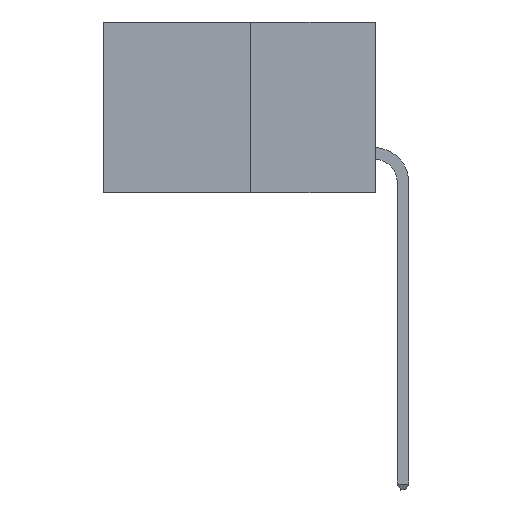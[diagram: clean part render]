
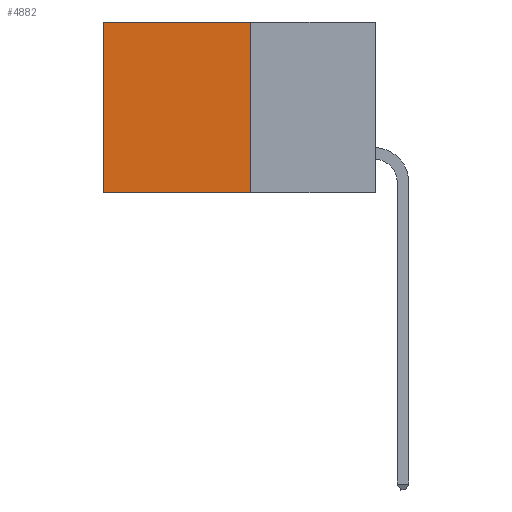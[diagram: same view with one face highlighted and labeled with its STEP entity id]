
A CAD part, left-side view. The second image highlights one B-rep face of the part: STEP entity #4882.
In plain terms, the highlighted planar face has unit normal (-1, 0, 0).
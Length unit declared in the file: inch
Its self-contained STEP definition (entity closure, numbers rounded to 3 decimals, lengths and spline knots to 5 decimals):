
#921 = CARTESIAN_POINT ( 'NONE',  ( 0.277, 0.27, -0.37 ) ) ;
#2353 = EDGE_LOOP ( 'NONE', ( #15523, #5587, #10960, #3823 ) ) ;
#2365 = CARTESIAN_POINT ( 'NONE',  ( 0.277, 0.27, -0.37 ) ) ;
#2819 = CARTESIAN_POINT ( 'NONE',  ( 0.277, 0.59, -0.37 ) ) ;
#2908 = VECTOR ( 'NONE', #8524, 39.37008 ) ;
#3176 = VECTOR ( 'NONE', #13594, 39.37008 ) ;
#3602 = LINE ( 'NONE', #15905, #3176 ) ;
#3663 = PLANE ( 'NONE',  #10400 ) ;
#3823 = ORIENTED_EDGE ( 'NONE', *, *, #6637, .T. ) ;
#3831 = CARTESIAN_POINT ( 'NONE',  ( 0.277, 0.27, -0.37 ) ) ;
#4474 = EDGE_CURVE ( 'NONE', #12852, #8963, #8583, .T. ) ;
#4534 = VECTOR ( 'NONE', #15949, 39.37008 ) ;
#4882 = ADVANCED_FACE ( 'NONE', ( #5289 ), #3663, .F. ) ;
#5234 = LINE ( 'NONE', #5258, #8136 ) ;
#5258 = CARTESIAN_POINT ( 'NONE',  ( 0.277, 0.27, -0.37 ) ) ;
#5289 = FACE_OUTER_BOUND ( 'NONE', #2353, .T. ) ;
#5308 = DIRECTION ( 'NONE',  ( 0., 0., -1. ) ) ;
#5587 = ORIENTED_EDGE ( 'NONE', *, *, #4474, .F. ) ;
#6637 = EDGE_CURVE ( 'NONE', #14142, #12935, #3602, .T. ) ;
#7026 = CARTESIAN_POINT ( 'NONE',  ( 0.277, 0.27, 0. ) ) ;
#7320 = CARTESIAN_POINT ( 'NONE',  ( 0.277, 0.59, -0.37 ) ) ;
#7426 = DIRECTION ( 'NONE',  ( 1., 0., 0. ) ) ;
#8136 = VECTOR ( 'NONE', #5308, 39.37008 ) ;
#8376 = EDGE_CURVE ( 'NONE', #12935, #8963, #12709, .T. ) ;
#8524 = DIRECTION ( 'NONE',  ( 0., 0., -1. ) ) ;
#8583 = LINE ( 'NONE', #3831, #4534 ) ;
#8963 = VERTEX_POINT ( 'NONE', #2819 ) ;
#10400 = AXIS2_PLACEMENT_3D ( 'NONE', #921, #7426, #15795 ) ;
#10960 = ORIENTED_EDGE ( 'NONE', *, *, #15887, .F. ) ;
#12709 = LINE ( 'NONE', #7320, #2908 ) ;
#12852 = VERTEX_POINT ( 'NONE', #2365 ) ;
#12935 = VERTEX_POINT ( 'NONE', #13558 ) ;
#13558 = CARTESIAN_POINT ( 'NONE',  ( 0.277, 0.59, 0. ) ) ;
#13594 = DIRECTION ( 'NONE',  ( 0., 1., 0. ) ) ;
#14142 = VERTEX_POINT ( 'NONE', #7026 ) ;
#15523 = ORIENTED_EDGE ( 'NONE', *, *, #8376, .T. ) ;
#15795 = DIRECTION ( 'NONE',  ( 0., 0., -1. ) ) ;
#15887 = EDGE_CURVE ( 'NONE', #14142, #12852, #5234, .T. ) ;
#15905 = CARTESIAN_POINT ( 'NONE',  ( 0.277, 0.27, 0. ) ) ;
#15949 = DIRECTION ( 'NONE',  ( 0., 1., 0. ) ) ;
